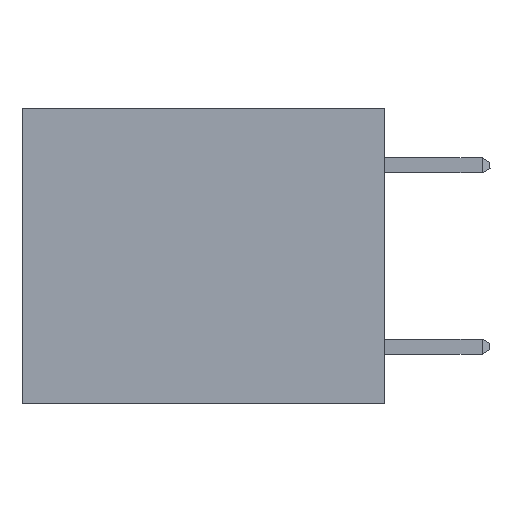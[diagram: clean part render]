
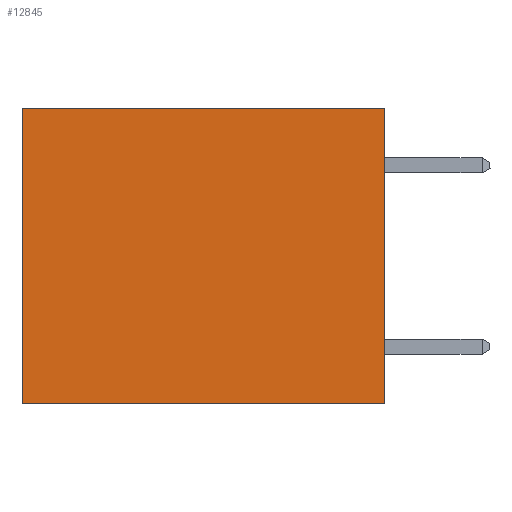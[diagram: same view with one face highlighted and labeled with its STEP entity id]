
A CAD part, left-side view. The second image highlights one B-rep face of the part: STEP entity #12845.
In plain terms, the highlighted planar face has unit normal (-1, 0, 0).
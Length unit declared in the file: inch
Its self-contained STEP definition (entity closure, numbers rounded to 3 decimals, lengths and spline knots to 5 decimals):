
#36 = DIRECTION ( 'NONE',  ( 0., 0., -1. ) ) ;
#221 = VERTEX_POINT ( 'NONE', #5688 ) ;
#886 = ORIENTED_EDGE ( 'NONE', *, *, #26855, .F. ) ;
#2675 = CARTESIAN_POINT ( 'NONE',  ( 0.3165, 0., -0.49 ) ) ;
#3605 = FACE_OUTER_BOUND ( 'NONE', #8518, .T. ) ;
#3878 = EDGE_CURVE ( 'NONE', #16987, #221, #23535, .T. ) ;
#3902 = CARTESIAN_POINT ( 'NONE',  ( 0.3165, 0., -0.49 ) ) ;
#5688 = CARTESIAN_POINT ( 'NONE',  ( 0.3165, 0.6, 0. ) ) ;
#6919 = LINE ( 'NONE', #3902, #14806 ) ;
#7807 = AXIS2_PLACEMENT_3D ( 'NONE', #12398, #12493, #28717 ) ;
#8281 = VECTOR ( 'NONE', #36, 39.37008 ) ;
#8518 = EDGE_LOOP ( 'NONE', ( #28732, #21355, #886, #28570 ) ) ;
#8757 = LINE ( 'NONE', #29423, #28636 ) ;
#10227 = CARTESIAN_POINT ( 'NONE',  ( 0.3165, 0., 0. ) ) ;
#12398 = CARTESIAN_POINT ( 'NONE',  ( 0.3165, 0., -0.49 ) ) ;
#12493 = DIRECTION ( 'NONE',  ( 1., 0., 0. ) ) ;
#12680 = CARTESIAN_POINT ( 'NONE',  ( 0.3165, 0., 0. ) ) ;
#12845 = ADVANCED_FACE ( 'NONE', ( #3605 ), #19407, .F. ) ;
#13763 = CARTESIAN_POINT ( 'NONE',  ( 0.3165, 0.6, -0.49 ) ) ;
#14806 = VECTOR ( 'NONE', #15509, 39.37008 ) ;
#15509 = DIRECTION ( 'NONE',  ( 0., 1., 0. ) ) ;
#15869 = CARTESIAN_POINT ( 'NONE',  ( 0.3165, 0., -0.49 ) ) ;
#16700 = EDGE_CURVE ( 'NONE', #23648, #29795, #6919, .T. ) ;
#16893 = LINE ( 'NONE', #2675, #8281 ) ;
#16987 = VERTEX_POINT ( 'NONE', #10227 ) ;
#17918 = DIRECTION ( 'NONE',  ( 0., 1., 0. ) ) ;
#18015 = VECTOR ( 'NONE', #17918, 39.37008 ) ;
#19407 = PLANE ( 'NONE',  #7807 ) ;
#21355 = ORIENTED_EDGE ( 'NONE', *, *, #16700, .F. ) ;
#21857 = EDGE_CURVE ( 'NONE', #221, #29795, #8757, .T. ) ;
#23535 = LINE ( 'NONE', #12680, #18015 ) ;
#23648 = VERTEX_POINT ( 'NONE', #15869 ) ;
#25294 = DIRECTION ( 'NONE',  ( 0., 0., -1. ) ) ;
#26855 = EDGE_CURVE ( 'NONE', #16987, #23648, #16893, .T. ) ;
#28570 = ORIENTED_EDGE ( 'NONE', *, *, #3878, .T. ) ;
#28636 = VECTOR ( 'NONE', #25294, 39.37008 ) ;
#28717 = DIRECTION ( 'NONE',  ( 0., 0., -1. ) ) ;
#28732 = ORIENTED_EDGE ( 'NONE', *, *, #21857, .T. ) ;
#29423 = CARTESIAN_POINT ( 'NONE',  ( 0.3165, 0.6, -0.49 ) ) ;
#29795 = VERTEX_POINT ( 'NONE', #13763 ) ;
